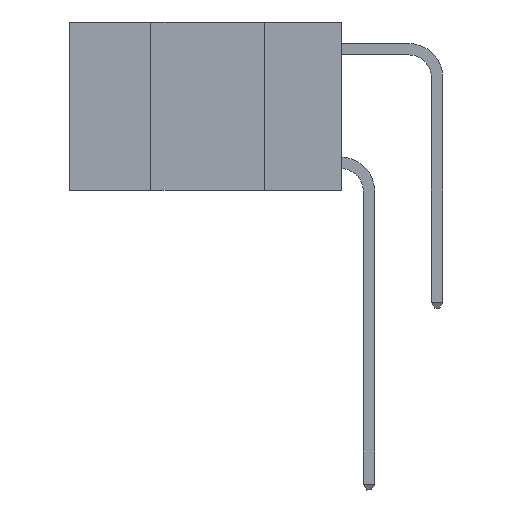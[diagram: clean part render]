
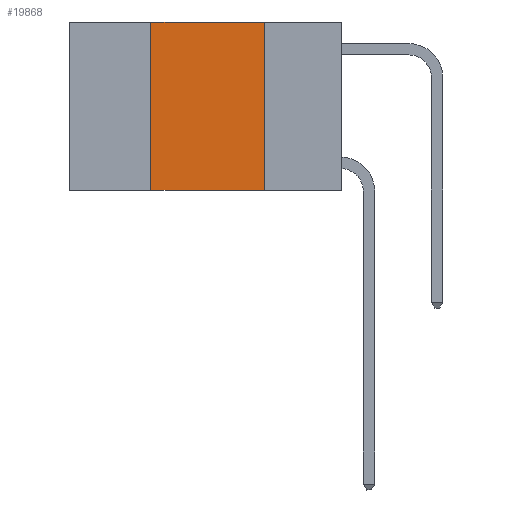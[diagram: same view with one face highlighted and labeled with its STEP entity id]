
A CAD part, left-side view. The second image highlights one B-rep face of the part: STEP entity #19868.
In plain terms, the highlighted planar face has unit normal (-1, 0, 0).
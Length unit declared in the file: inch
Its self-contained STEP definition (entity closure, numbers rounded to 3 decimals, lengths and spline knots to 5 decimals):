
#1301 = VERTEX_POINT ( 'NONE', #4436 ) ;
#1317 = EDGE_CURVE ( 'NONE', #17009, #1301, #14127, .T. ) ;
#2792 = EDGE_CURVE ( 'NONE', #28620, #29170, #5285, .T. ) ;
#2981 = CARTESIAN_POINT ( 'NONE',  ( 0., 0.42, 0. ) ) ;
#3169 = CARTESIAN_POINT ( 'NONE',  ( 0., 0.17, 0. ) ) ;
#3322 = CARTESIAN_POINT ( 'NONE',  ( 0., 0.17, -0.37 ) ) ;
#3338 = EDGE_CURVE ( 'NONE', #1301, #29170, #21075, .T. ) ;
#3776 = AXIS2_PLACEMENT_3D ( 'NONE', #16720, #7067, #23920 ) ;
#4436 = CARTESIAN_POINT ( 'NONE',  ( 0., 0.17, 0. ) ) ;
#4540 = CARTESIAN_POINT ( 'NONE',  ( 0., 0.6, 0. ) ) ;
#4669 = ORIENTED_EDGE ( 'NONE', *, *, #1317, .F. ) ;
#5285 = LINE ( 'NONE', #12805, #30139 ) ;
#5393 = ORIENTED_EDGE ( 'NONE', *, *, #2792, .T. ) ;
#7067 = DIRECTION ( 'NONE',  ( 1., 0., 0. ) ) ;
#7364 = EDGE_LOOP ( 'NONE', ( #28744, #4669, #30254, #5393 ) ) ;
#7655 = VECTOR ( 'NONE', #28613, 39.37008 ) ;
#8236 = VECTOR ( 'NONE', #17602, 39.37008 ) ;
#9442 = PLANE ( 'NONE',  #3776 ) ;
#10969 = CARTESIAN_POINT ( 'NONE',  ( 0., 0.42, 0. ) ) ;
#12805 = CARTESIAN_POINT ( 'NONE',  ( 0., 0.6, -0.37 ) ) ;
#13405 = DIRECTION ( 'NONE',  ( 0., 0., 1. ) ) ;
#14127 = LINE ( 'NONE', #4540, #7655 ) ;
#16704 = VECTOR ( 'NONE', #13405, 39.37008 ) ;
#16720 = CARTESIAN_POINT ( 'NONE',  ( 0., 0.6, 0. ) ) ;
#17009 = VERTEX_POINT ( 'NONE', #2981 ) ;
#17602 = DIRECTION ( 'NONE',  ( 0., 0., -1. ) ) ;
#18199 = LINE ( 'NONE', #10969, #16704 ) ;
#18918 = EDGE_CURVE ( 'NONE', #28620, #17009, #18199, .T. ) ;
#19868 = ADVANCED_FACE ( 'NONE', ( #21843 ), #9442, .F. ) ;
#21075 = LINE ( 'NONE', #3169, #8236 ) ;
#21843 = FACE_OUTER_BOUND ( 'NONE', #7364, .T. ) ;
#23920 = DIRECTION ( 'NONE',  ( 0., 0., -1. ) ) ;
#27139 = DIRECTION ( 'NONE',  ( 0., -1., 0. ) ) ;
#27713 = CARTESIAN_POINT ( 'NONE',  ( 0., 0.42, -0.37 ) ) ;
#28613 = DIRECTION ( 'NONE',  ( 0., -1., 0. ) ) ;
#28620 = VERTEX_POINT ( 'NONE', #27713 ) ;
#28744 = ORIENTED_EDGE ( 'NONE', *, *, #3338, .F. ) ;
#29170 = VERTEX_POINT ( 'NONE', #3322 ) ;
#30139 = VECTOR ( 'NONE', #27139, 39.37008 ) ;
#30254 = ORIENTED_EDGE ( 'NONE', *, *, #18918, .F. ) ;
